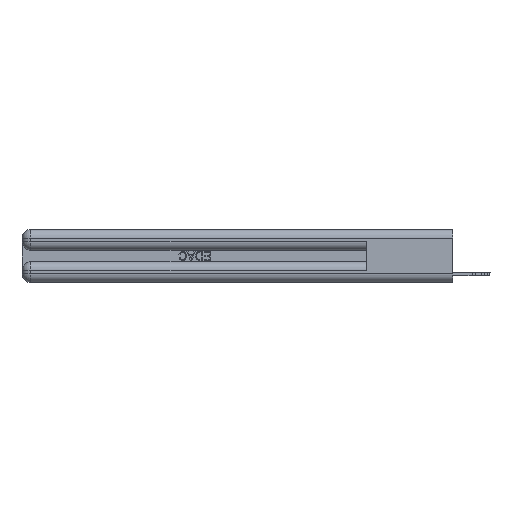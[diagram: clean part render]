
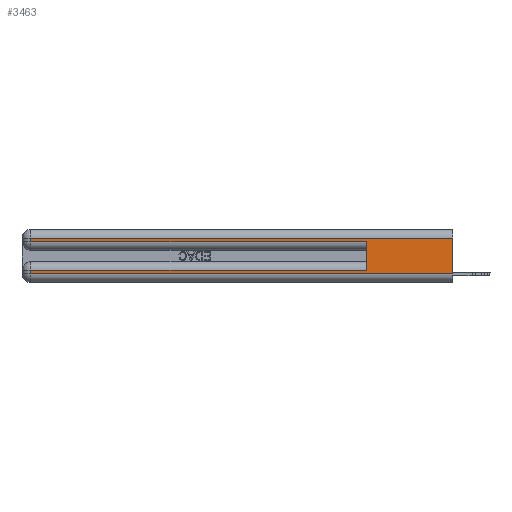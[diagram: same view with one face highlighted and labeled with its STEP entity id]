
A CAD part, left-side view. The second image highlights one B-rep face of the part: STEP entity #3463.
In plain terms, the highlighted planar face has unit normal (-1, 0, 0).
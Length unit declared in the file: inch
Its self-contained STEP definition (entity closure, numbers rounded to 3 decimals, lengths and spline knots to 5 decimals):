
#76 = ORIENTED_EDGE ( 'NONE', *, *, #30150, .T. ) ;
#1695 = VECTOR ( 'NONE', #28407, 39.37008 ) ;
#2123 = DIRECTION ( 'NONE',  ( 1., 0., 0. ) ) ;
#2314 = CARTESIAN_POINT ( 'NONE',  ( 0., 2.94, 0.37 ) ) ;
#2858 = VECTOR ( 'NONE', #18824, 39.37008 ) ;
#2892 = CARTESIAN_POINT ( 'NONE',  ( 0., 0., 0.06 ) ) ;
#2897 = AXIS2_PLACEMENT_3D ( 'NONE', #23406, #2123, #7270 ) ;
#3191 = VECTOR ( 'NONE', #4370, 39.37008 ) ;
#3463 = ADVANCED_FACE ( 'NONE', ( #7110 ), #14229, .F. ) ;
#4186 = CARTESIAN_POINT ( 'NONE',  ( 0., 0., 0.31 ) ) ;
#4370 = DIRECTION ( 'NONE',  ( 0., 0., -1. ) ) ;
#5333 = VERTEX_POINT ( 'NONE', #12220 ) ;
#5572 = CARTESIAN_POINT ( 'NONE',  ( 0., 2.94, 0.06 ) ) ;
#6558 = LINE ( 'NONE', #11369, #27571 ) ;
#7059 = CARTESIAN_POINT ( 'NONE',  ( 0., 0., 0.37 ) ) ;
#7110 = FACE_OUTER_BOUND ( 'NONE', #9524, .T. ) ;
#7270 = DIRECTION ( 'NONE',  ( 0., 0., -1. ) ) ;
#7986 = LINE ( 'NONE', #23805, #11781 ) ;
#8163 = CARTESIAN_POINT ( 'NONE',  ( 0., 2.94, 0.085 ) ) ;
#8424 = VERTEX_POINT ( 'NONE', #18889 ) ;
#8479 = CARTESIAN_POINT ( 'NONE',  ( 0., 0., 0.085 ) ) ;
#9524 = EDGE_LOOP ( 'NONE', ( #16707, #11718, #13302, #12943, #25438, #25797, #76, #17574 ) ) ;
#11369 = CARTESIAN_POINT ( 'NONE',  ( 0., 0., 0.285 ) ) ;
#11506 = CARTESIAN_POINT ( 'NONE',  ( 0., 0., 0.06 ) ) ;
#11718 = ORIENTED_EDGE ( 'NONE', *, *, #22426, .T. ) ;
#11781 = VECTOR ( 'NONE', #11998, 39.37008 ) ;
#11998 = DIRECTION ( 'NONE',  ( 0., 0., -1. ) ) ;
#12029 = EDGE_CURVE ( 'NONE', #24075, #12224, #23211, .T. ) ;
#12030 = CARTESIAN_POINT ( 'NONE',  ( 0., 0., 0.31 ) ) ;
#12220 = CARTESIAN_POINT ( 'NONE',  ( 0., 0.6, 0.285 ) ) ;
#12224 = VERTEX_POINT ( 'NONE', #2892 ) ;
#12320 = CARTESIAN_POINT ( 'NONE',  ( 0., 0.6, 0.145 ) ) ;
#12726 = VERTEX_POINT ( 'NONE', #15363 ) ;
#12943 = ORIENTED_EDGE ( 'NONE', *, *, #18195, .T. ) ;
#13229 = DIRECTION ( 'NONE',  ( 0., 1., 0. ) ) ;
#13302 = ORIENTED_EDGE ( 'NONE', *, *, #24737, .T. ) ;
#13667 = LINE ( 'NONE', #11506, #26078 ) ;
#14093 = LINE ( 'NONE', #2314, #3191 ) ;
#14229 = PLANE ( 'NONE',  #2897 ) ;
#15286 = CARTESIAN_POINT ( 'NONE',  ( 0., 0.6, 0.085 ) ) ;
#15363 = CARTESIAN_POINT ( 'NONE',  ( 0., 2.94, 0.285 ) ) ;
#15455 = EDGE_CURVE ( 'NONE', #17615, #5333, #21459, .T. ) ;
#16510 = VERTEX_POINT ( 'NONE', #5572 ) ;
#16707 = ORIENTED_EDGE ( 'NONE', *, *, #12029, .F. ) ;
#17574 = ORIENTED_EDGE ( 'NONE', *, *, #23310, .T. ) ;
#17615 = VERTEX_POINT ( 'NONE', #15286 ) ;
#17684 = VERTEX_POINT ( 'NONE', #8163 ) ;
#18010 = DIRECTION ( 'NONE',  ( 0., -1., 0. ) ) ;
#18195 = EDGE_CURVE ( 'NONE', #12726, #5333, #6558, .T. ) ;
#18824 = DIRECTION ( 'NONE',  ( 0., 0., -1. ) ) ;
#18889 = CARTESIAN_POINT ( 'NONE',  ( 0., 2.94, 0.31 ) ) ;
#21097 = VECTOR ( 'NONE', #23858, 39.37008 ) ;
#21459 = LINE ( 'NONE', #12320, #1695 ) ;
#22426 = EDGE_CURVE ( 'NONE', #24075, #8424, #25423, .T. ) ;
#23211 = LINE ( 'NONE', #7059, #2858 ) ;
#23310 = EDGE_CURVE ( 'NONE', #16510, #12224, #13667, .T. ) ;
#23406 = CARTESIAN_POINT ( 'NONE',  ( 0., 0., 0.37 ) ) ;
#23805 = CARTESIAN_POINT ( 'NONE',  ( 0., 2.94, 0.37 ) ) ;
#23858 = DIRECTION ( 'NONE',  ( 0., 1., 0. ) ) ;
#24075 = VERTEX_POINT ( 'NONE', #12030 ) ;
#24737 = EDGE_CURVE ( 'NONE', #8424, #12726, #7986, .T. ) ;
#25423 = LINE ( 'NONE', #4186, #21097 ) ;
#25438 = ORIENTED_EDGE ( 'NONE', *, *, #15455, .F. ) ;
#25797 = ORIENTED_EDGE ( 'NONE', *, *, #26820, .T. ) ;
#26078 = VECTOR ( 'NONE', #18010, 39.37008 ) ;
#26820 = EDGE_CURVE ( 'NONE', #17615, #17684, #29678, .T. ) ;
#27571 = VECTOR ( 'NONE', #28223, 39.37008 ) ;
#27733 = VECTOR ( 'NONE', #13229, 39.37008 ) ;
#28223 = DIRECTION ( 'NONE',  ( 0., -1., 0. ) ) ;
#28407 = DIRECTION ( 'NONE',  ( 0., 0., 1. ) ) ;
#29678 = LINE ( 'NONE', #8479, #27733 ) ;
#30150 = EDGE_CURVE ( 'NONE', #17684, #16510, #14093, .T. ) ;
